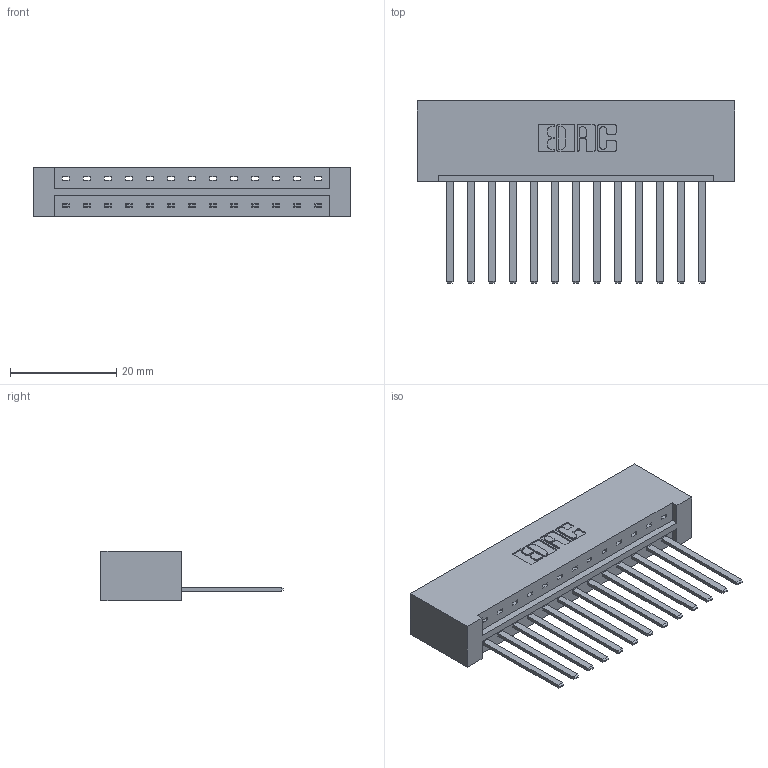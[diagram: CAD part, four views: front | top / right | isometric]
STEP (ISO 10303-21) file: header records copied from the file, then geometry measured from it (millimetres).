
FILE_DESCRIPTION (( 'STEP AP203' ), '1' );
FILE_NAME ('333-013-544-101.STEP', '2018-08-01T01:33:55', ( '' ), ( '' ), 'SwSTEP 2.0', 'SolidWorks 2016', '' );
FILE_SCHEMA (( 'CONFIG_CONTROL_DESIGN' ));
Length unit declared in the file: inch
Products named in the file (3): 333 Part_Lugless; 345-292-001_345-293-144; 333-013-544-101
Assembly tree (14 placements, depth 2):
  333-013-544-101
    333 Part_Lugless
    345-292-001_345-293-144  x13
Bounding box: 59.77 x 34.3 x 9.4 mm (x, y, z)
Volume: 6528.1 mm3; surface area: 7319.5 mm2
Topology: 14 solids, 14 shells, 782 faces, 2341 edges, 1542 vertices
Faces by surface type: plane 560, cylinder 222
Entity records: 11237 total; most frequent: CARTESIAN_POINT 1949, ORIENTED_EDGE 1898, DIRECTION 1691, EDGE_CURVE 949, VECTOR 833, LINE 833, VERTEX_POINT 630, AXIS2_PLACEMENT_3D 429
